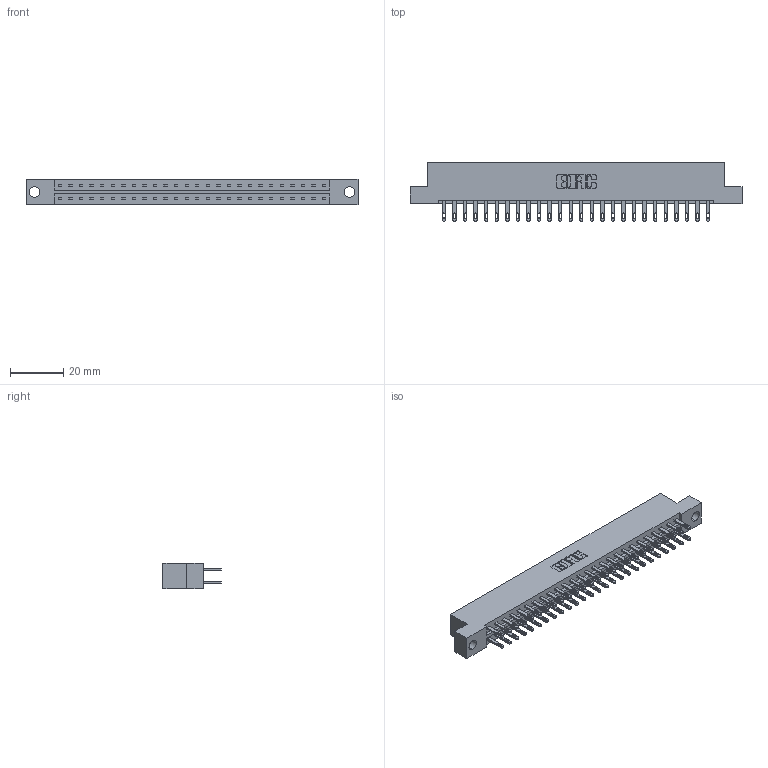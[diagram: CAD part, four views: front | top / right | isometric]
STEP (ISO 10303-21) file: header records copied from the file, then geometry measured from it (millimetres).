
FILE_DESCRIPTION (( 'STEP AP203' ), '1' );
FILE_NAME ('333-052-500-204.STEP', '2018-08-04T01:43:54', ( '' ), ( '' ), 'SwSTEP 2.0', 'SolidWorks 2016', '' );
FILE_SCHEMA (( 'CONFIG_CONTROL_DESIGN' ));
Length unit declared in the file: inch
Products named in the file (3): 333 Part_Flush - .156 Dia - TH; 345-292-001_345-293-100; 333-052-500-204
Assembly tree (53 placements, depth 2):
  333-052-500-204
    333 Part_Flush - .156 Dia - TH
    345-292-001_345-293-100  x52
Bounding box: 124.56 x 21.85 x 9.4 mm (x, y, z)
Volume: 12638.4 mm3; surface area: 15141.5 mm2
Topology: 53 solids, 53 shells, 2610 faces, 7955 edges, 5302 vertices
Faces by surface type: plane 1630, cylinder 980
Entity records: 18729 total; most frequent: CARTESIAN_POINT 3122, ORIENTED_EDGE 3058, DIRECTION 2697, EDGE_CURVE 1529, LINE 1397, VECTOR 1397, VERTEX_POINT 1018, AXIS2_PLACEMENT_3D 650
